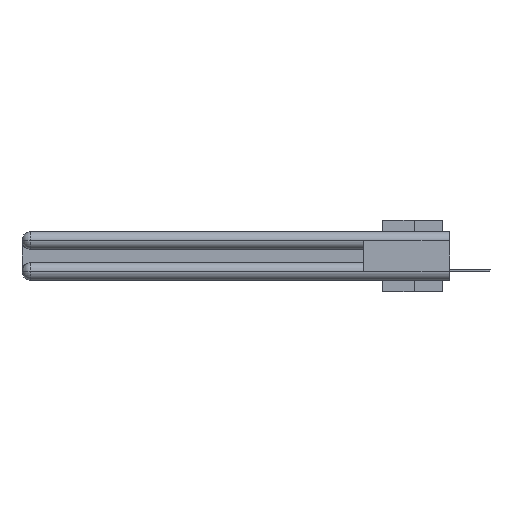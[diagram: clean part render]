
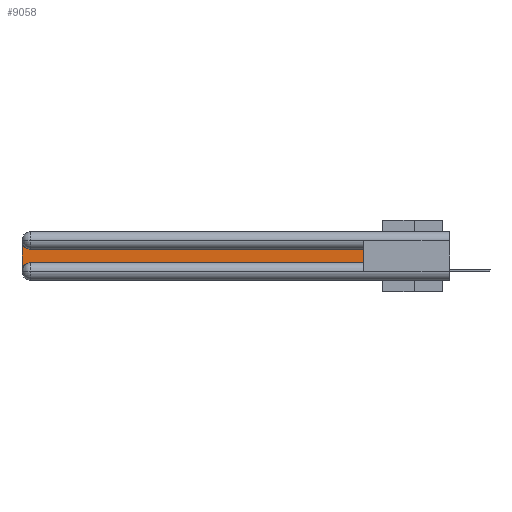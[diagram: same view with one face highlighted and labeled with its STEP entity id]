
A CAD part, left-side view. The second image highlights one B-rep face of the part: STEP entity #9058.
In plain terms, the highlighted planar face has unit normal (-1, 0, 0).
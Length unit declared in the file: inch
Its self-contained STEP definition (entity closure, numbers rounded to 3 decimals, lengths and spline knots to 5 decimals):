
#64 = CIRCLE ( 'NONE', #16460, 0.06 ) ;
#949 = CARTESIAN_POINT ( 'NONE',  ( 0.075, 0.6, -0.1225 ) ) ;
#1025 = ORIENTED_EDGE ( 'NONE', *, *, #21888, .T. ) ;
#1166 = DIRECTION ( 'NONE',  ( 0., 0., -1. ) ) ;
#1370 = CARTESIAN_POINT ( 'NONE',  ( 0.075, 3., -0.1225 ) ) ;
#2155 = VERTEX_POINT ( 'NONE', #33712 ) ;
#2636 = ORIENTED_EDGE ( 'NONE', *, *, #10507, .T. ) ;
#2953 = CARTESIAN_POINT ( 'NONE',  ( 0.075, 0.6, -0.1225 ) ) ;
#3841 = VERTEX_POINT ( 'NONE', #12378 ) ;
#4730 = VECTOR ( 'NONE', #26514, 39.37008 ) ;
#5535 = FACE_OUTER_BOUND ( 'NONE', #28577, .T. ) ;
#5847 = CARTESIAN_POINT ( 'NONE',  ( 0.075, 2.94, -0.1225 ) ) ;
#6948 = CARTESIAN_POINT ( 'NONE',  ( 0.075, 2.94, -0.2175 ) ) ;
#7633 = LINE ( 'NONE', #33496, #33796 ) ;
#8832 = EDGE_CURVE ( 'NONE', #3841, #13340, #13131, .T. ) ;
#9058 = ADVANCED_FACE ( 'NONE', ( #5535 ), #28386, .F. ) ;
#9133 = ORIENTED_EDGE ( 'NONE', *, *, #26026, .T. ) ;
#9322 = CARTESIAN_POINT ( 'NONE',  ( 0.075, 2.94, -0.2775 ) ) ;
#9616 = ORIENTED_EDGE ( 'NONE', *, *, #8832, .T. ) ;
#10070 = ORIENTED_EDGE ( 'NONE', *, *, #16045, .T. ) ;
#10507 = EDGE_CURVE ( 'NONE', #29904, #3841, #21490, .T. ) ;
#10750 = ORIENTED_EDGE ( 'NONE', *, *, #22509, .T. ) ;
#11239 = AXIS2_PLACEMENT_3D ( 'NONE', #28738, #28502, #25887 ) ;
#12231 = DIRECTION ( 'NONE',  ( 0., 0., -1. ) ) ;
#12378 = CARTESIAN_POINT ( 'NONE',  ( 0.075, 0.6, -0.2175 ) ) ;
#13131 = LINE ( 'NONE', #32071, #4730 ) ;
#13340 = VERTEX_POINT ( 'NONE', #949 ) ;
#16045 = EDGE_CURVE ( 'NONE', #2155, #29904, #64, .T. ) ;
#16460 = AXIS2_PLACEMENT_3D ( 'NONE', #9322, #28191, #30893 ) ;
#16915 = CIRCLE ( 'NONE', #11239, 0.06 ) ;
#17185 = VERTEX_POINT ( 'NONE', #31391 ) ;
#19363 = DIRECTION ( 'NONE',  ( 0., 1., 0. ) ) ;
#21490 = LINE ( 'NONE', #26197, #28636 ) ;
#21888 = EDGE_CURVE ( 'NONE', #17185, #2155, #7633, .T. ) ;
#22509 = EDGE_CURVE ( 'NONE', #13340, #24608, #28282, .T. ) ;
#23231 = DIRECTION ( 'NONE',  ( 1., 0., 0. ) ) ;
#24253 = AXIS2_PLACEMENT_3D ( 'NONE', #1370, #23231, #12231 ) ;
#24608 = VERTEX_POINT ( 'NONE', #5847 ) ;
#24892 = VECTOR ( 'NONE', #19363, 39.37008 ) ;
#25887 = DIRECTION ( 'NONE',  ( 0., 0., -1. ) ) ;
#26026 = EDGE_CURVE ( 'NONE', #24608, #17185, #16915, .T. ) ;
#26078 = DIRECTION ( 'NONE',  ( 0., -1., 0. ) ) ;
#26197 = CARTESIAN_POINT ( 'NONE',  ( 0.075, 0.6, -0.2175 ) ) ;
#26514 = DIRECTION ( 'NONE',  ( 0., 0., 1. ) ) ;
#28191 = DIRECTION ( 'NONE',  ( 1., 0., 0. ) ) ;
#28282 = LINE ( 'NONE', #2953, #24892 ) ;
#28386 = PLANE ( 'NONE',  #24253 ) ;
#28502 = DIRECTION ( 'NONE',  ( 1., 0., 0. ) ) ;
#28577 = EDGE_LOOP ( 'NONE', ( #10750, #9133, #1025, #10070, #2636, #9616 ) ) ;
#28636 = VECTOR ( 'NONE', #26078, 39.37008 ) ;
#28738 = CARTESIAN_POINT ( 'NONE',  ( 0.075, 2.94, -0.0625 ) ) ;
#29904 = VERTEX_POINT ( 'NONE', #6948 ) ;
#30893 = DIRECTION ( 'NONE',  ( 0., 0., -1. ) ) ;
#31391 = CARTESIAN_POINT ( 'NONE',  ( 0.075, 3., -0.0625 ) ) ;
#32071 = CARTESIAN_POINT ( 'NONE',  ( 0.075, 0.6, -0.2175 ) ) ;
#33496 = CARTESIAN_POINT ( 'NONE',  ( 0.075, 3., -0.2175 ) ) ;
#33712 = CARTESIAN_POINT ( 'NONE',  ( 0.075, 3., -0.2775 ) ) ;
#33796 = VECTOR ( 'NONE', #1166, 39.37008 ) ;
